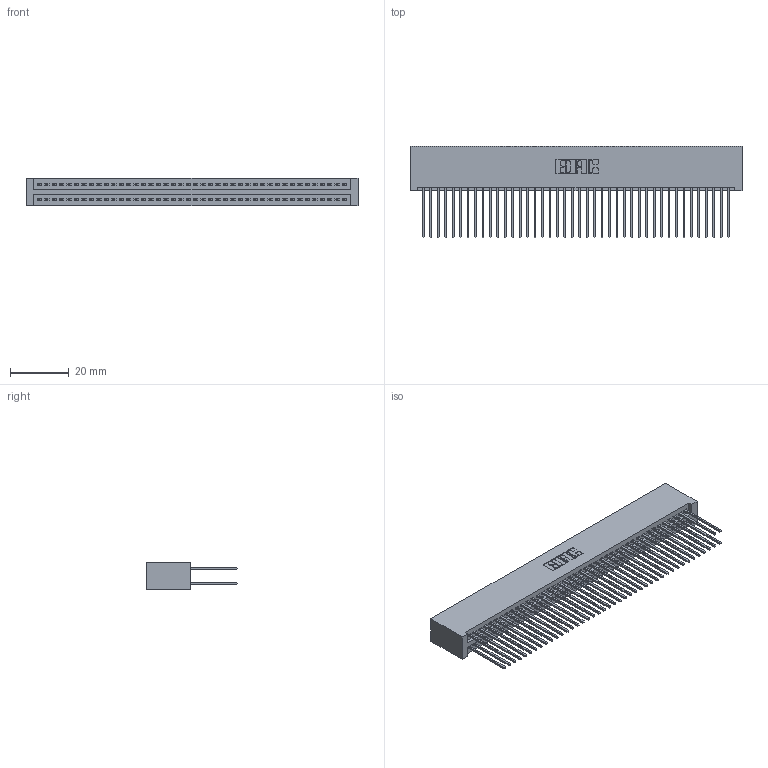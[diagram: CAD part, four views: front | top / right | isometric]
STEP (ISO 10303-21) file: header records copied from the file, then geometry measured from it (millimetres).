
FILE_DESCRIPTION (( 'STEP AP203' ), '1' );
FILE_NAME ('345-084-542-201.STEP', '2018-10-04T01:57:27', ( '' ), ( '' ), 'SwSTEP 2.0', 'SolidWorks 2016', '' );
FILE_SCHEMA (( 'CONFIG_CONTROL_DESIGN' ));
Length unit declared in the file: inch
Products named in the file (3): 345-084-542-201; 345 Part_No Mounting Lugs; 345-292-001_345-293-142
Assembly tree (85 placements, depth 2):
  345-084-542-201
    345 Part_No Mounting Lugs
    345-292-001_345-293-142  x84
Bounding box: 113.28 x 31.29 x 9.4 mm (x, y, z)
Volume: 12012 mm3; surface area: 19889 mm2
Topology: 85 solids, 85 shells, 4318 faces, 12833 edges, 8442 vertices
Faces by surface type: plane 2848, cylinder 1470
Entity records: 32695 total; most frequent: CARTESIAN_POINT 5480, ORIENTED_EDGE 5414, DIRECTION 4827, EDGE_CURVE 2707, VECTOR 2415, LINE 2415, VERTEX_POINT 1802, AXIS2_PLACEMENT_3D 1206
